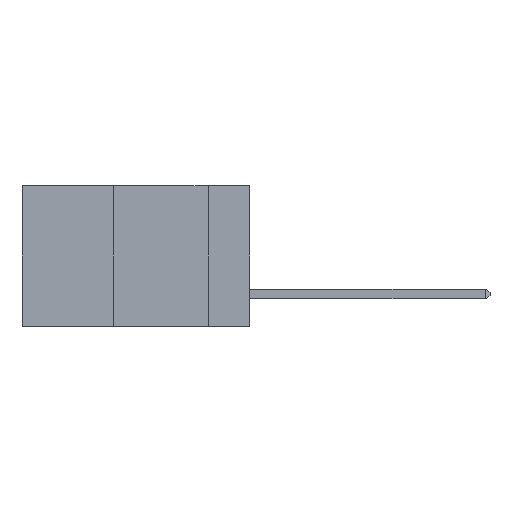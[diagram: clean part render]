
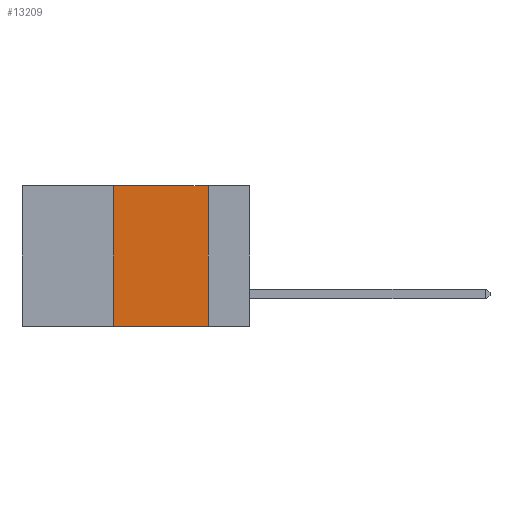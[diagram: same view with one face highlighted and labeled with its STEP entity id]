
A CAD part, left-side view. The second image highlights one B-rep face of the part: STEP entity #13209.
In plain terms, the highlighted planar face has unit normal (-1, 0, 0).
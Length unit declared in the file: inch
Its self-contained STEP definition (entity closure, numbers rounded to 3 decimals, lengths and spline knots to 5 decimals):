
#878 = VECTOR ( 'NONE', #28943, 39.37008 ) ;
#993 = ORIENTED_EDGE ( 'NONE', *, *, #3360, .F. ) ;
#1552 = LINE ( 'NONE', #6266, #7658 ) ;
#2020 = VERTEX_POINT ( 'NONE', #19677 ) ;
#2944 = ORIENTED_EDGE ( 'NONE', *, *, #26743, .F. ) ;
#3360 = EDGE_CURVE ( 'NONE', #16511, #6368, #22954, .T. ) ;
#4854 = CARTESIAN_POINT ( 'NONE',  ( 0., 0.6, 0. ) ) ;
#6266 = CARTESIAN_POINT ( 'NONE',  ( 0., 0.6, 0. ) ) ;
#6368 = VERTEX_POINT ( 'NONE', #23400 ) ;
#7482 = DIRECTION ( 'NONE',  ( 0., 0., -1. ) ) ;
#7658 = VECTOR ( 'NONE', #28605, 39.37008 ) ;
#8220 = DIRECTION ( 'NONE',  ( 0., 0., 1. ) ) ;
#8493 = VERTEX_POINT ( 'NONE', #29849 ) ;
#8793 = AXIS2_PLACEMENT_3D ( 'NONE', #4854, #22323, #7482 ) ;
#9067 = ORIENTED_EDGE ( 'NONE', *, *, #10687, .T. ) ;
#10687 = EDGE_CURVE ( 'NONE', #16511, #8493, #18614, .T. ) ;
#11686 = CARTESIAN_POINT ( 'NONE',  ( 0., 0.6, -0.37 ) ) ;
#11836 = CARTESIAN_POINT ( 'NONE',  ( 0., 0.11, 0. ) ) ;
#12861 = CARTESIAN_POINT ( 'NONE',  ( 0., 0.36, -0.37 ) ) ;
#13209 = ADVANCED_FACE ( 'NONE', ( #15358 ), #32103, .F. ) ;
#14321 = DIRECTION ( 'NONE',  ( 0., 0., -1. ) ) ;
#14864 = EDGE_LOOP ( 'NONE', ( #2944, #20299, #993, #9067 ) ) ;
#15358 = FACE_OUTER_BOUND ( 'NONE', #14864, .T. ) ;
#15734 = VECTOR ( 'NONE', #14321, 39.37008 ) ;
#16511 = VERTEX_POINT ( 'NONE', #12861 ) ;
#18614 = LINE ( 'NONE', #11686, #878 ) ;
#19677 = CARTESIAN_POINT ( 'NONE',  ( 0., 0.11, 0. ) ) ;
#20299 = ORIENTED_EDGE ( 'NONE', *, *, #25940, .F. ) ;
#21389 = VECTOR ( 'NONE', #8220, 39.37008 ) ;
#22323 = DIRECTION ( 'NONE',  ( 1., 0., 0. ) ) ;
#22330 = LINE ( 'NONE', #11836, #15734 ) ;
#22954 = LINE ( 'NONE', #30335, #21389 ) ;
#23400 = CARTESIAN_POINT ( 'NONE',  ( 0., 0.36, 0. ) ) ;
#25940 = EDGE_CURVE ( 'NONE', #6368, #2020, #1552, .T. ) ;
#26743 = EDGE_CURVE ( 'NONE', #2020, #8493, #22330, .T. ) ;
#28605 = DIRECTION ( 'NONE',  ( 0., -1., 0. ) ) ;
#28943 = DIRECTION ( 'NONE',  ( 0., -1., 0. ) ) ;
#29849 = CARTESIAN_POINT ( 'NONE',  ( 0., 0.11, -0.37 ) ) ;
#30335 = CARTESIAN_POINT ( 'NONE',  ( 0., 0.36, 0. ) ) ;
#32103 = PLANE ( 'NONE',  #8793 ) ;
